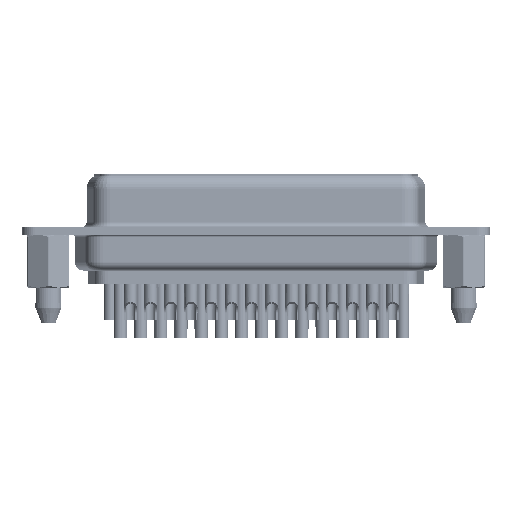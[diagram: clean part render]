
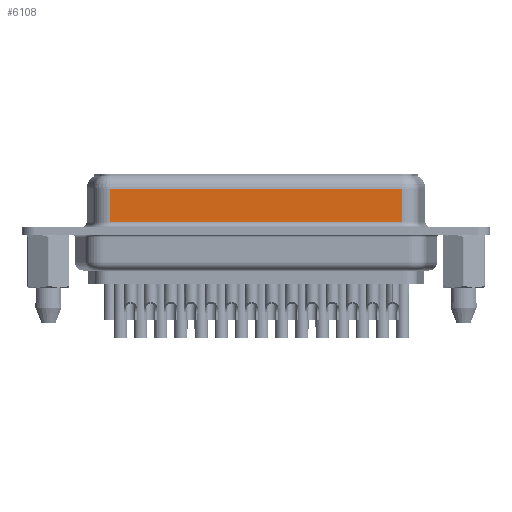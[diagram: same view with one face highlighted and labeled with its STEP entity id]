
A CAD part, front view. The second image highlights one B-rep face of the part: STEP entity #6108.
In plain terms, the highlighted planar face has unit normal (0, -1, 0).
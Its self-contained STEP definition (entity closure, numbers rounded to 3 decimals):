
#1495 = ORIENTED_EDGE ( 'NONE', *, *, #22702, .T. ) ;
#1995 = CARTESIAN_POINT ( 'NONE',  ( 7.008, -3.95, 6.45 ) ) ;
#3176 = CARTESIAN_POINT ( 'NONE',  ( 40.032, -3.95, 0.95 ) ) ;
#3897 = AXIS2_PLACEMENT_3D ( 'NONE', #28495, #36614, #11151 ) ;
#4353 = LINE ( 'NONE', #29842, #7907 ) ;
#5836 = EDGE_CURVE ( 'NONE', #30355, #7764, #8760, .T. ) ;
#6108 = ADVANCED_FACE ( 'NONE', ( #27926 ), #24924, .F. ) ;
#6493 = CARTESIAN_POINT ( 'NONE',  ( 7.008, -3.95, 0.95 ) ) ;
#7074 = LINE ( 'NONE', #13112, #29303 ) ;
#7764 = VERTEX_POINT ( 'NONE', #3176 ) ;
#7907 = VECTOR ( 'NONE', #35857, 1000. ) ;
#8760 = LINE ( 'NONE', #26644, #36856 ) ;
#9399 = CARTESIAN_POINT ( 'NONE',  ( 40.032, -3.95, 4.7 ) ) ;
#11151 = DIRECTION ( 'NONE',  ( 0., 0., 1. ) ) ;
#12335 = DIRECTION ( 'NONE',  ( 0., 0., -1. ) ) ;
#13112 = CARTESIAN_POINT ( 'NONE',  ( 40.032, -3.95, 0.95 ) ) ;
#13534 = DIRECTION ( 'NONE',  ( 0., 0., -1. ) ) ;
#17001 = EDGE_CURVE ( 'NONE', #31345, #34164, #27824, .T. ) ;
#17333 = EDGE_CURVE ( 'NONE', #34164, #7764, #7074, .T. ) ;
#18317 = ORIENTED_EDGE ( 'NONE', *, *, #17333, .T. ) ;
#19217 = CARTESIAN_POINT ( 'NONE',  ( 7.008, -3.95, 4.7 ) ) ;
#22702 = EDGE_CURVE ( 'NONE', #30355, #31345, #4353, .T. ) ;
#24924 = PLANE ( 'NONE',  #3897 ) ;
#26265 = ORIENTED_EDGE ( 'NONE', *, *, #17001, .T. ) ;
#26644 = CARTESIAN_POINT ( 'NONE',  ( 40.032, -3.95, 6.45 ) ) ;
#27824 = LINE ( 'NONE', #1995, #34667 ) ;
#27926 = FACE_OUTER_BOUND ( 'NONE', #31491, .T. ) ;
#28495 = CARTESIAN_POINT ( 'NONE',  ( 40.032, -3.95, 6.45 ) ) ;
#29303 = VECTOR ( 'NONE', #35161, 1000. ) ;
#29842 = CARTESIAN_POINT ( 'NONE',  ( 40.032, -3.95, 4.7 ) ) ;
#30355 = VERTEX_POINT ( 'NONE', #9399 ) ;
#31345 = VERTEX_POINT ( 'NONE', #19217 ) ;
#31491 = EDGE_LOOP ( 'NONE', ( #34121, #1495, #26265, #18317 ) ) ;
#34121 = ORIENTED_EDGE ( 'NONE', *, *, #5836, .F. ) ;
#34164 = VERTEX_POINT ( 'NONE', #6493 ) ;
#34667 = VECTOR ( 'NONE', #13534, 1000. ) ;
#35161 = DIRECTION ( 'NONE',  ( 1., 0., 0. ) ) ;
#35857 = DIRECTION ( 'NONE',  ( -1., 0., 0. ) ) ;
#36614 = DIRECTION ( 'NONE',  ( 0., 1., 0. ) ) ;
#36856 = VECTOR ( 'NONE', #12335, 1000. ) ;
